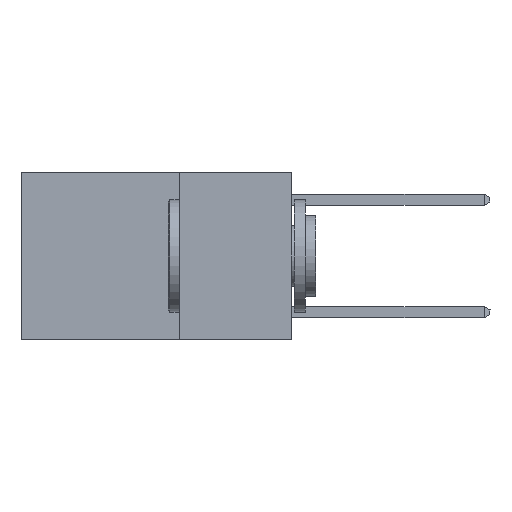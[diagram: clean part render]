
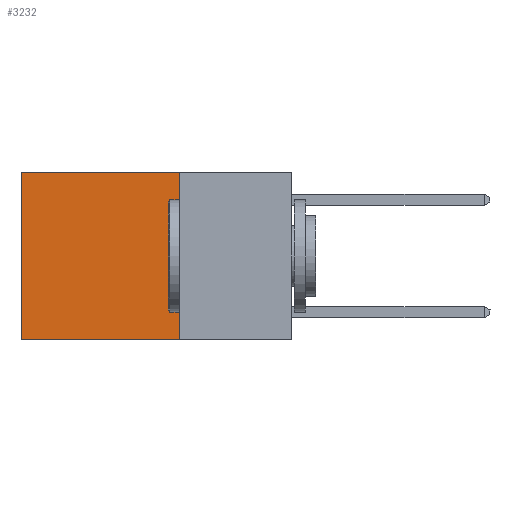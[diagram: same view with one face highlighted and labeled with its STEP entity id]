
A CAD part, left-side view. The second image highlights one B-rep face of the part: STEP entity #3232.
In plain terms, the highlighted planar face has unit normal (-1, 0, 0).
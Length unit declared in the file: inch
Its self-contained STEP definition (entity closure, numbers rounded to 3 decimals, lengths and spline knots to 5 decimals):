
#845 = VERTEX_POINT ( 'NONE', #12626 ) ;
#1089 = DIRECTION ( 'NONE',  ( 0., 0., -1. ) ) ;
#1328 = ORIENTED_EDGE ( 'NONE', *, *, #15050, .T. ) ;
#1375 = ORIENTED_EDGE ( 'NONE', *, *, #15406, .F. ) ;
#2430 = VECTOR ( 'NONE', #9413, 39.37008 ) ;
#2560 = ORIENTED_EDGE ( 'NONE', *, *, #24105, .F. ) ;
#2652 = AXIS2_PLACEMENT_3D ( 'NONE', #17502, #5239, #19634 ) ;
#3215 = ORIENTED_EDGE ( 'NONE', *, *, #26475, .T. ) ;
#3232 = ADVANCED_FACE ( 'NONE', ( #5141 ), #15452, .F. ) ;
#3315 = VERTEX_POINT ( 'NONE', #25784 ) ;
#4043 = LINE ( 'NONE', #17670, #24529 ) ;
#5097 = LINE ( 'NONE', #18718, #25489 ) ;
#5141 = FACE_OUTER_BOUND ( 'NONE', #18488, .T. ) ;
#5239 = DIRECTION ( 'NONE',  ( 1., 0., 0. ) ) ;
#5744 = CARTESIAN_POINT ( 'NONE',  ( 0.2625, 0.25, 0. ) ) ;
#8498 = LINE ( 'NONE', #5744, #13891 ) ;
#9413 = DIRECTION ( 'NONE',  ( 0., 0., -1. ) ) ;
#12626 = CARTESIAN_POINT ( 'NONE',  ( 0.2625, 0.25, 0. ) ) ;
#13269 = VERTEX_POINT ( 'NONE', #14505 ) ;
#13891 = VECTOR ( 'NONE', #20157, 39.37008 ) ;
#14505 = CARTESIAN_POINT ( 'NONE',  ( 0.2625, 0.6, -0.37 ) ) ;
#15050 = EDGE_CURVE ( 'NONE', #21801, #13269, #18278, .T. ) ;
#15406 = EDGE_CURVE ( 'NONE', #3315, #13269, #5097, .T. ) ;
#15452 = PLANE ( 'NONE',  #2652 ) ;
#17502 = CARTESIAN_POINT ( 'NONE',  ( 0.2625, 0.25, 0. ) ) ;
#17670 = CARTESIAN_POINT ( 'NONE',  ( 0.2625, 0.25, 0. ) ) ;
#18053 = CARTESIAN_POINT ( 'NONE',  ( 0.2625, 0.6, 0. ) ) ;
#18278 = LINE ( 'NONE', #25649, #2430 ) ;
#18488 = EDGE_LOOP ( 'NONE', ( #1328, #1375, #2560, #3215 ) ) ;
#18718 = CARTESIAN_POINT ( 'NONE',  ( 0.2625, 0.25, -0.37 ) ) ;
#19634 = DIRECTION ( 'NONE',  ( 0., 0., -1. ) ) ;
#20157 = DIRECTION ( 'NONE',  ( 0., 1., 0. ) ) ;
#21801 = VERTEX_POINT ( 'NONE', #18053 ) ;
#22865 = DIRECTION ( 'NONE',  ( 0., 1., 0. ) ) ;
#24105 = EDGE_CURVE ( 'NONE', #845, #3315, #4043, .T. ) ;
#24529 = VECTOR ( 'NONE', #1089, 39.37008 ) ;
#25489 = VECTOR ( 'NONE', #22865, 39.37008 ) ;
#25649 = CARTESIAN_POINT ( 'NONE',  ( 0.2625, 0.6, 0. ) ) ;
#25784 = CARTESIAN_POINT ( 'NONE',  ( 0.2625, 0.25, -0.37 ) ) ;
#26475 = EDGE_CURVE ( 'NONE', #845, #21801, #8498, .T. ) ;
